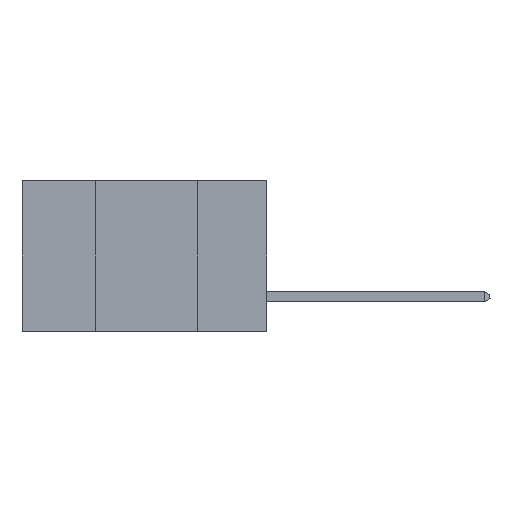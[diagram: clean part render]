
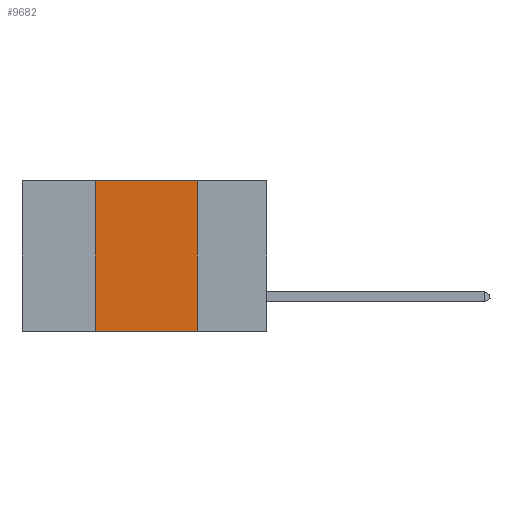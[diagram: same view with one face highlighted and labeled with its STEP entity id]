
A CAD part, left-side view. The second image highlights one B-rep face of the part: STEP entity #9682.
In plain terms, the highlighted planar face has unit normal (-1, 0, 0).
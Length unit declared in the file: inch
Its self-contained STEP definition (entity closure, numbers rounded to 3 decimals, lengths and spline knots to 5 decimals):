
#254 = VECTOR ( 'NONE', #3886, 39.37008 ) ;
#534 = DIRECTION ( 'NONE',  ( 1., 0., 0. ) ) ;
#1826 = DIRECTION ( 'NONE',  ( 0., 0., -1. ) ) ;
#2169 = LINE ( 'NONE', #8578, #17523 ) ;
#2509 = ORIENTED_EDGE ( 'NONE', *, *, #11385, .F. ) ;
#2659 = ORIENTED_EDGE ( 'NONE', *, *, #7904, .T. ) ;
#2773 = EDGE_CURVE ( 'NONE', #9668, #9952, #6139, .T. ) ;
#3711 = EDGE_CURVE ( 'NONE', #15834, #10946, #14717, .T. ) ;
#3823 = CARTESIAN_POINT ( 'NONE',  ( 0., 0.6, 0. ) ) ;
#3886 = DIRECTION ( 'NONE',  ( 0., -1., 0. ) ) ;
#3942 = PLANE ( 'NONE',  #14924 ) ;
#3969 = CARTESIAN_POINT ( 'NONE',  ( 0., 0.17, 0. ) ) ;
#4744 = FACE_OUTER_BOUND ( 'NONE', #17756, .T. ) ;
#5115 = CARTESIAN_POINT ( 'NONE',  ( 0., 0.42, -0.37 ) ) ;
#6139 = LINE ( 'NONE', #3969, #10986 ) ;
#6782 = DIRECTION ( 'NONE',  ( 0., 0., 1. ) ) ;
#7079 = CARTESIAN_POINT ( 'NONE',  ( 0., 0.17, 0. ) ) ;
#7120 = CARTESIAN_POINT ( 'NONE',  ( 0., 0.17, -0.37 ) ) ;
#7904 = EDGE_CURVE ( 'NONE', #15834, #9952, #2169, .T. ) ;
#8578 = CARTESIAN_POINT ( 'NONE',  ( 0., 0.6, -0.37 ) ) ;
#9150 = CARTESIAN_POINT ( 'NONE',  ( 0., 0.42, 0. ) ) ;
#9209 = ORIENTED_EDGE ( 'NONE', *, *, #2773, .F. ) ;
#9668 = VERTEX_POINT ( 'NONE', #7079 ) ;
#9682 = ADVANCED_FACE ( 'NONE', ( #4744 ), #3942, .F. ) ;
#9930 = CARTESIAN_POINT ( 'NONE',  ( 0., 0.6, 0. ) ) ;
#9952 = VERTEX_POINT ( 'NONE', #7120 ) ;
#10201 = ORIENTED_EDGE ( 'NONE', *, *, #3711, .F. ) ;
#10518 = VECTOR ( 'NONE', #6782, 39.37008 ) ;
#10779 = CARTESIAN_POINT ( 'NONE',  ( 0., 0.42, 0. ) ) ;
#10946 = VERTEX_POINT ( 'NONE', #9150 ) ;
#10986 = VECTOR ( 'NONE', #16588, 39.37008 ) ;
#11385 = EDGE_CURVE ( 'NONE', #10946, #9668, #15227, .T. ) ;
#12679 = DIRECTION ( 'NONE',  ( 0., -1., 0. ) ) ;
#14717 = LINE ( 'NONE', #10779, #10518 ) ;
#14924 = AXIS2_PLACEMENT_3D ( 'NONE', #9930, #534, #1826 ) ;
#15227 = LINE ( 'NONE', #3823, #254 ) ;
#15834 = VERTEX_POINT ( 'NONE', #5115 ) ;
#16588 = DIRECTION ( 'NONE',  ( 0., 0., -1. ) ) ;
#17523 = VECTOR ( 'NONE', #12679, 39.37008 ) ;
#17756 = EDGE_LOOP ( 'NONE', ( #9209, #2509, #10201, #2659 ) ) ;
